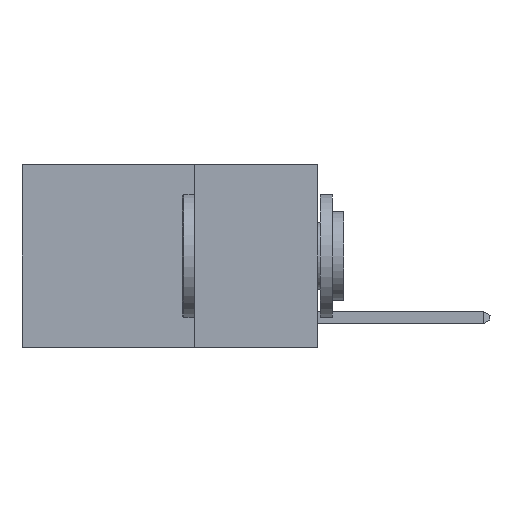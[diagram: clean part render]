
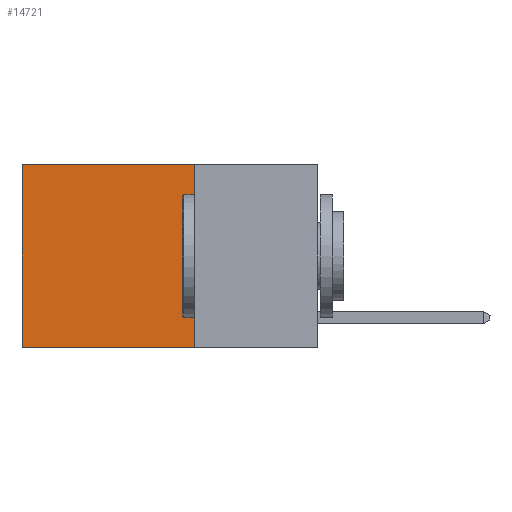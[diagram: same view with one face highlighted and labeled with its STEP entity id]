
A CAD part, left-side view. The second image highlights one B-rep face of the part: STEP entity #14721.
In plain terms, the highlighted planar face has unit normal (-1, 0, 0).
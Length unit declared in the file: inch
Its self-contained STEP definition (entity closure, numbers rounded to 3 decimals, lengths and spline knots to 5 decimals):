
#94 = DIRECTION ( 'NONE',  ( 0., 1., 0. ) ) ;
#585 = CARTESIAN_POINT ( 'NONE',  ( 0.2625, 0.6, 0. ) ) ;
#919 = DIRECTION ( 'NONE',  ( 0., 1., 0. ) ) ;
#1261 = DIRECTION ( 'NONE',  ( 1., 0., 0. ) ) ;
#1957 = VECTOR ( 'NONE', #94, 39.37008 ) ;
#1993 = VECTOR ( 'NONE', #15524, 39.37008 ) ;
#3214 = ORIENTED_EDGE ( 'NONE', *, *, #7639, .T. ) ;
#5616 = CARTESIAN_POINT ( 'NONE',  ( 0.2625, 0.25, -0.37 ) ) ;
#5650 = ORIENTED_EDGE ( 'NONE', *, *, #15183, .F. ) ;
#6470 = VECTOR ( 'NONE', #15247, 39.37008 ) ;
#6703 = ORIENTED_EDGE ( 'NONE', *, *, #10642, .F. ) ;
#7188 = PLANE ( 'NONE',  #14793 ) ;
#7619 = LINE ( 'NONE', #13447, #9167 ) ;
#7639 = EDGE_CURVE ( 'NONE', #11402, #18316, #7619, .T. ) ;
#7808 = EDGE_LOOP ( 'NONE', ( #10463, #5650, #6703, #3214 ) ) ;
#8049 = CARTESIAN_POINT ( 'NONE',  ( 0.2625, 0.6, 0. ) ) ;
#8508 = FACE_OUTER_BOUND ( 'NONE', #7808, .T. ) ;
#9167 = VECTOR ( 'NONE', #919, 39.37008 ) ;
#9373 = CARTESIAN_POINT ( 'NONE',  ( 0.2625, 0.6, -0.37 ) ) ;
#10463 = ORIENTED_EDGE ( 'NONE', *, *, #17830, .T. ) ;
#10585 = LINE ( 'NONE', #16445, #1957 ) ;
#10642 = EDGE_CURVE ( 'NONE', #11402, #11784, #16589, .T. ) ;
#10829 = CARTESIAN_POINT ( 'NONE',  ( 0.2625, 0.25, 0. ) ) ;
#11368 = CARTESIAN_POINT ( 'NONE',  ( 0.2625, 0.25, 0. ) ) ;
#11402 = VERTEX_POINT ( 'NONE', #13756 ) ;
#11784 = VERTEX_POINT ( 'NONE', #5616 ) ;
#12323 = VERTEX_POINT ( 'NONE', #9373 ) ;
#13447 = CARTESIAN_POINT ( 'NONE',  ( 0.2625, 0.25, 0. ) ) ;
#13756 = CARTESIAN_POINT ( 'NONE',  ( 0.2625, 0.25, 0. ) ) ;
#14167 = LINE ( 'NONE', #8049, #1993 ) ;
#14721 = ADVANCED_FACE ( 'NONE', ( #8508 ), #7188, .F. ) ;
#14793 = AXIS2_PLACEMENT_3D ( 'NONE', #11368, #1261, #15902 ) ;
#15183 = EDGE_CURVE ( 'NONE', #11784, #12323, #10585, .T. ) ;
#15247 = DIRECTION ( 'NONE',  ( 0., 0., -1. ) ) ;
#15524 = DIRECTION ( 'NONE',  ( 0., 0., -1. ) ) ;
#15902 = DIRECTION ( 'NONE',  ( 0., 0., -1. ) ) ;
#16445 = CARTESIAN_POINT ( 'NONE',  ( 0.2625, 0.25, -0.37 ) ) ;
#16589 = LINE ( 'NONE', #10829, #6470 ) ;
#17830 = EDGE_CURVE ( 'NONE', #18316, #12323, #14167, .T. ) ;
#18316 = VERTEX_POINT ( 'NONE', #585 ) ;
